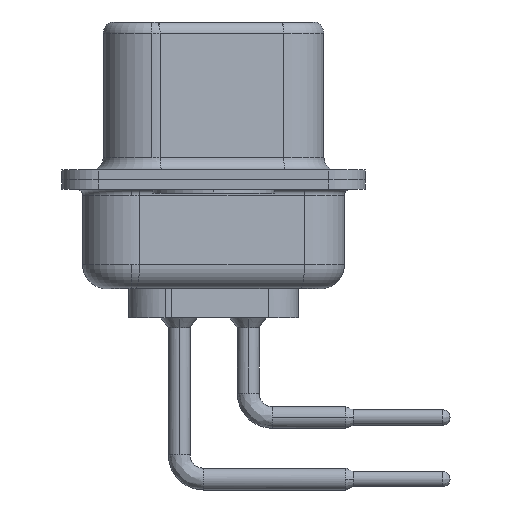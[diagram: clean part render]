
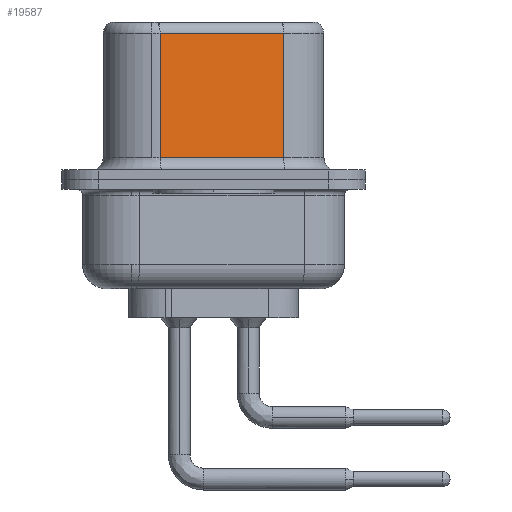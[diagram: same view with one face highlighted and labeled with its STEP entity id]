
A CAD part, left-side view. The second image highlights one B-rep face of the part: STEP entity #19587.
In plain terms, the highlighted planar face has unit normal (-0.985, -0.174, 0).
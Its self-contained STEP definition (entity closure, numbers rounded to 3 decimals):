
#53 = CARTESIAN_POINT ( 'NONE',  ( 4.58, -2.897, 6.02 ) ) ;
#872 = VECTOR ( 'NONE', #13478, 1000. ) ;
#1232 = CARTESIAN_POINT ( 'NONE',  ( 3.68, 2.203, 6.02 ) ) ;
#1281 = VECTOR ( 'NONE', #8958, 1000. ) ;
#1614 = AXIS2_PLACEMENT_3D ( 'NONE', #22891, #25087, #12167 ) ;
#3161 = ORIENTED_EDGE ( 'NONE', *, *, #20176, .T. ) ;
#4777 = EDGE_CURVE ( 'NONE', #9587, #11137, #16380, .T. ) ;
#5484 = DIRECTION ( 'NONE',  ( 0., 0., -1. ) ) ;
#6302 = ORIENTED_EDGE ( 'NONE', *, *, #4777, .F. ) ;
#6950 = LINE ( 'NONE', #12137, #12126 ) ;
#7132 = CARTESIAN_POINT ( 'NONE',  ( 3.68, 2.203, 0.9 ) ) ;
#7376 = LINE ( 'NONE', #21895, #1281 ) ;
#8234 = ORIENTED_EDGE ( 'NONE', *, *, #13227, .T. ) ;
#8958 = DIRECTION ( 'NONE',  ( 0.174, -0.985, 0. ) ) ;
#9587 = VERTEX_POINT ( 'NONE', #19128 ) ;
#9982 = PLANE ( 'NONE',  #1614 ) ;
#10574 = VECTOR ( 'NONE', #28031, 1000. ) ;
#11137 = VERTEX_POINT ( 'NONE', #23182 ) ;
#12126 = VECTOR ( 'NONE', #5484, 1000. ) ;
#12137 = CARTESIAN_POINT ( 'NONE',  ( 3.68, 2.203, 6.52 ) ) ;
#12167 = DIRECTION ( 'NONE',  ( -0.174, 0.985, 0. ) ) ;
#12536 = EDGE_CURVE ( 'NONE', #24355, #11137, #7376, .T. ) ;
#12931 = ORIENTED_EDGE ( 'NONE', *, *, #12536, .T. ) ;
#13006 = CARTESIAN_POINT ( 'NONE',  ( 4.58, -2.897, 6.52 ) ) ;
#13227 = EDGE_CURVE ( 'NONE', #9587, #22217, #24276, .T. ) ;
#13478 = DIRECTION ( 'NONE',  ( -0.174, 0.985, 0. ) ) ;
#15652 = EDGE_LOOP ( 'NONE', ( #6302, #8234, #3161, #12931 ) ) ;
#16380 = LINE ( 'NONE', #13006, #10574 ) ;
#19128 = CARTESIAN_POINT ( 'NONE',  ( 4.58, -2.897, 6.02 ) ) ;
#19587 = ADVANCED_FACE ( 'NONE', ( #19890 ), #9982, .F. ) ;
#19890 = FACE_OUTER_BOUND ( 'NONE', #15652, .T. ) ;
#20176 = EDGE_CURVE ( 'NONE', #22217, #24355, #6950, .T. ) ;
#21895 = CARTESIAN_POINT ( 'NONE',  ( 4.58, -2.897, 0.9 ) ) ;
#22217 = VERTEX_POINT ( 'NONE', #1232 ) ;
#22891 = CARTESIAN_POINT ( 'NONE',  ( 4.58, -2.897, 6.52 ) ) ;
#23182 = CARTESIAN_POINT ( 'NONE',  ( 4.58, -2.897, 0.9 ) ) ;
#24276 = LINE ( 'NONE', #53, #872 ) ;
#24355 = VERTEX_POINT ( 'NONE', #7132 ) ;
#25087 = DIRECTION ( 'NONE',  ( 0.985, 0.174, 0. ) ) ;
#28031 = DIRECTION ( 'NONE',  ( 0., 0., -1. ) ) ;
